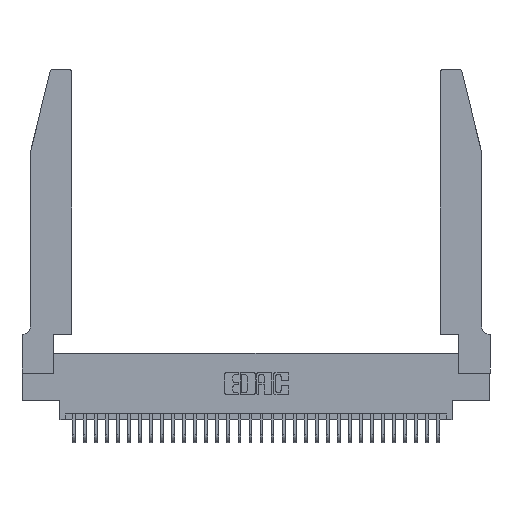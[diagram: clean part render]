
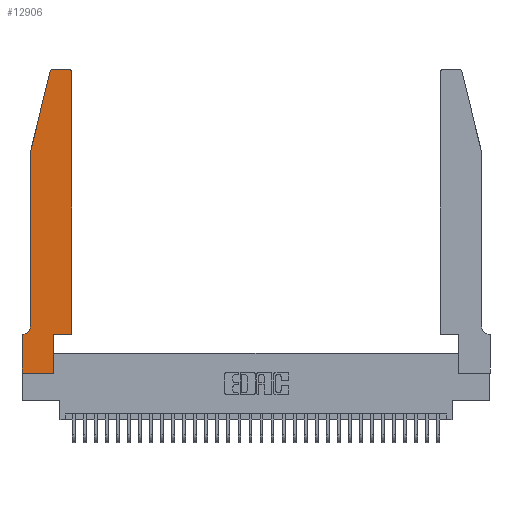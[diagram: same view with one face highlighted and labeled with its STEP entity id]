
A CAD part, top view. The second image highlights one B-rep face of the part: STEP entity #12906.
In plain terms, the highlighted planar face has unit normal (0, 0, 1).
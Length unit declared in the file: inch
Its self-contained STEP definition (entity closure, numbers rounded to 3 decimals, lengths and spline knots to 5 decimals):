
#100 = CARTESIAN_POINT ( 'NONE',  ( 0., 0., 0.37 ) ) ;
#483 = ORIENTED_EDGE ( 'NONE', *, *, #10885, .T. ) ;
#1708 = ORIENTED_EDGE ( 'NONE', *, *, #18758, .T. ) ;
#1712 = CARTESIAN_POINT ( 'NONE',  ( 0., 0., 0.37 ) ) ;
#1976 = VECTOR ( 'NONE', #15647, 39.37008 ) ;
#2194 = VERTEX_POINT ( 'NONE', #19306 ) ;
#2786 = LINE ( 'NONE', #8092, #14014 ) ;
#3056 = ORIENTED_EDGE ( 'NONE', *, *, #9239, .T. ) ;
#3841 = VERTEX_POINT ( 'NONE', #9479 ) ;
#4585 = ORIENTED_EDGE ( 'NONE', *, *, #24579, .T. ) ;
#4782 = AXIS2_PLACEMENT_3D ( 'NONE', #13715, #29688, #21488 ) ;
#4790 = ORIENTED_EDGE ( 'NONE', *, *, #8335, .T. ) ;
#4834 = VERTEX_POINT ( 'NONE', #13871 ) ;
#4869 = PLANE ( 'NONE',  #12304 ) ;
#4973 = CARTESIAN_POINT ( 'NONE',  ( 0., 0.35, 0.37 ) ) ;
#5071 = CARTESIAN_POINT ( 'NONE',  ( 0.0755, 0.35, 0.37 ) ) ;
#5328 = LINE ( 'NONE', #18245, #18576 ) ;
#5451 = DIRECTION ( 'NONE',  ( 0., 1., 0. ) ) ;
#5560 = ORIENTED_EDGE ( 'NONE', *, *, #13677, .T. ) ;
#5928 = EDGE_CURVE ( 'NONE', #4834, #14161, #2786, .T. ) ;
#6035 = EDGE_CURVE ( 'NONE', #13258, #4834, #9853, .T. ) ;
#6407 = AXIS2_PLACEMENT_3D ( 'NONE', #7086, #17550, #12203 ) ;
#6743 = ORIENTED_EDGE ( 'NONE', *, *, #17718, .T. ) ;
#7086 = CARTESIAN_POINT ( 'NONE',  ( 0.284, 2.72, 0.37 ) ) ;
#7091 = CARTESIAN_POINT ( 'NONE',  ( 0.4505, 0.35, 0.37 ) ) ;
#7308 = CARTESIAN_POINT ( 'NONE',  ( 0., 0.35, 0.37 ) ) ;
#8092 = CARTESIAN_POINT ( 'NONE',  ( 0.2605, 2.75, 0.37 ) ) ;
#8335 = EDGE_CURVE ( 'NONE', #22696, #25335, #5328, .T. ) ;
#9239 = EDGE_CURVE ( 'NONE', #25866, #18439, #31846, .T. ) ;
#9294 = EDGE_CURVE ( 'NONE', #17986, #2194, #12413, .T. ) ;
#9311 = CIRCLE ( 'NONE', #6407, 0.03 ) ;
#9479 = CARTESIAN_POINT ( 'NONE',  ( 0.0755, 0.42, 0.37 ) ) ;
#9753 = EDGE_CURVE ( 'NONE', #3841, #27666, #23589, .T. ) ;
#9853 = CIRCLE ( 'NONE', #24681, 0.03 ) ;
#9892 = LINE ( 'NONE', #31781, #1976 ) ;
#10885 = EDGE_CURVE ( 'NONE', #25335, #3841, #9892, .T. ) ;
#11465 = ORIENTED_EDGE ( 'NONE', *, *, #5928, .T. ) ;
#11801 = CARTESIAN_POINT ( 'NONE',  ( 0.4505, 0.35, 0.37 ) ) ;
#12203 = DIRECTION ( 'NONE',  ( 1., 0., 0. ) ) ;
#12304 = AXIS2_PLACEMENT_3D ( 'NONE', #7308, #12535, #23076 ) ;
#12413 = LINE ( 'NONE', #1712, #18644 ) ;
#12535 = DIRECTION ( 'NONE',  ( 0., 0., 1. ) ) ;
#12906 = ADVANCED_FACE ( 'NONE', ( #31659 ), #4869, .T. ) ;
#13166 = DIRECTION ( 'NONE',  ( -0.239, -0.971, 0. ) ) ;
#13258 = VERTEX_POINT ( 'NONE', #26895 ) ;
#13347 = CARTESIAN_POINT ( 'NONE',  ( 0.4505, 0.35, 0.37 ) ) ;
#13487 = DIRECTION ( 'NONE',  ( -1., 0., 0. ) ) ;
#13556 = DIRECTION ( 'NONE',  ( 0., 0., 1. ) ) ;
#13677 = EDGE_CURVE ( 'NONE', #27666, #20175, #26714, .T. ) ;
#13715 = CARTESIAN_POINT ( 'NONE',  ( 0.0055, 0.42, 0.37 ) ) ;
#13834 = VECTOR ( 'NONE', #5451, 39.37008 ) ;
#13871 = CARTESIAN_POINT ( 'NONE',  ( 0.4205, 2.75, 0.37 ) ) ;
#14014 = VECTOR ( 'NONE', #13487, 39.37008 ) ;
#14161 = VERTEX_POINT ( 'NONE', #23033 ) ;
#14289 = DIRECTION ( 'NONE',  ( 0., -1., 0. ) ) ;
#15647 = DIRECTION ( 'NONE',  ( 0., -1., 0. ) ) ;
#15763 = DIRECTION ( 'NONE',  ( 1., 0., 0. ) ) ;
#16779 = CARTESIAN_POINT ( 'NONE',  ( 0.0055, 0.35, 0.37 ) ) ;
#17139 = DIRECTION ( 'NONE',  ( 0., 1., 0. ) ) ;
#17550 = DIRECTION ( 'NONE',  ( 0., 0., 1. ) ) ;
#17718 = EDGE_CURVE ( 'NONE', #14161, #22696, #9311, .T. ) ;
#17986 = VERTEX_POINT ( 'NONE', #100 ) ;
#18245 = CARTESIAN_POINT ( 'NONE',  ( 0.0755, 2., 0.37 ) ) ;
#18439 = VERTEX_POINT ( 'NONE', #13347 ) ;
#18576 = VECTOR ( 'NONE', #13166, 39.37008 ) ;
#18644 = VECTOR ( 'NONE', #20310, 39.37008 ) ;
#18758 = EDGE_CURVE ( 'NONE', #2194, #25866, #31203, .T. ) ;
#19120 = CARTESIAN_POINT ( 'NONE',  ( 0.4205, 2.72, 0.37 ) ) ;
#19306 = CARTESIAN_POINT ( 'NONE',  ( 0.2865, 0., 0.37 ) ) ;
#19434 = CARTESIAN_POINT ( 'NONE',  ( 0.2865, 0.35, 0.37 ) ) ;
#19487 = EDGE_CURVE ( 'NONE', #18439, #13258, #29941, .T. ) ;
#20142 = CARTESIAN_POINT ( 'NONE',  ( 0.2865, 0.35, 0.37 ) ) ;
#20175 = VERTEX_POINT ( 'NONE', #4973 ) ;
#20310 = DIRECTION ( 'NONE',  ( 1., 0., 0. ) ) ;
#21488 = DIRECTION ( 'NONE',  ( -1., 0., 0. ) ) ;
#21637 = ORIENTED_EDGE ( 'NONE', *, *, #9753, .T. ) ;
#21796 = DIRECTION ( 'NONE',  ( 1., 0., 0. ) ) ;
#21961 = CARTESIAN_POINT ( 'NONE',  ( 0.25487, 2.72718, 0.37 ) ) ;
#22696 = VERTEX_POINT ( 'NONE', #21961 ) ;
#22981 = VECTOR ( 'NONE', #17139, 39.37008 ) ;
#23033 = CARTESIAN_POINT ( 'NONE',  ( 0.284, 2.75, 0.37 ) ) ;
#23076 = DIRECTION ( 'NONE',  ( 1., 0., 0. ) ) ;
#23108 = ORIENTED_EDGE ( 'NONE', *, *, #19487, .T. ) ;
#23302 = ORIENTED_EDGE ( 'NONE', *, *, #9294, .T. ) ;
#23589 = CIRCLE ( 'NONE', #4782, 0.07 ) ;
#24364 = EDGE_LOOP ( 'NONE', ( #11465, #6743, #4790, #483, #21637, #5560, #4585, #23302, #1708, #3056, #23108, #31982 ) ) ;
#24579 = EDGE_CURVE ( 'NONE', #20175, #17986, #31220, .T. ) ;
#24656 = CARTESIAN_POINT ( 'NONE',  ( 0.0755, 2., 0.37 ) ) ;
#24681 = AXIS2_PLACEMENT_3D ( 'NONE', #19120, #13556, #21796 ) ;
#25335 = VERTEX_POINT ( 'NONE', #24656 ) ;
#25866 = VERTEX_POINT ( 'NONE', #19434 ) ;
#26714 = LINE ( 'NONE', #5071, #30790 ) ;
#26895 = CARTESIAN_POINT ( 'NONE',  ( 0.4505, 2.72, 0.37 ) ) ;
#27666 = VERTEX_POINT ( 'NONE', #16779 ) ;
#29600 = VECTOR ( 'NONE', #14289, 39.37008 ) ;
#29688 = DIRECTION ( 'NONE',  ( 0., 0., -1. ) ) ;
#29827 = VECTOR ( 'NONE', #15763, 39.37008 ) ;
#29941 = LINE ( 'NONE', #11801, #13834 ) ;
#30790 = VECTOR ( 'NONE', #30993, 39.37008 ) ;
#30993 = DIRECTION ( 'NONE',  ( -1., 0., 0. ) ) ;
#31203 = LINE ( 'NONE', #20142, #22981 ) ;
#31220 = LINE ( 'NONE', #31848, #29600 ) ;
#31659 = FACE_OUTER_BOUND ( 'NONE', #24364, .T. ) ;
#31781 = CARTESIAN_POINT ( 'NONE',  ( 0.0755, 2., 0.37 ) ) ;
#31846 = LINE ( 'NONE', #7091, #29827 ) ;
#31848 = CARTESIAN_POINT ( 'NONE',  ( 0., 0., 0.37 ) ) ;
#31982 = ORIENTED_EDGE ( 'NONE', *, *, #6035, .T. ) ;
